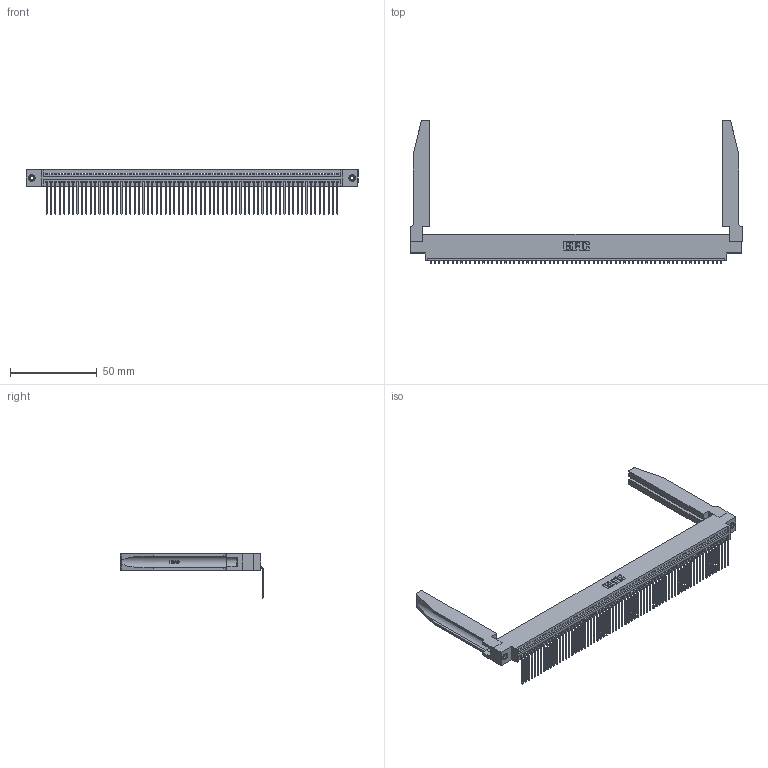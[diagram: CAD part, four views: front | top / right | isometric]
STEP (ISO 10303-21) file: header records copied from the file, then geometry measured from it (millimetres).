
FILE_DESCRIPTION (( 'STEP AP203' ), '1' );
FILE_NAME ('345-067-559-678.STEP', '2019-10-12T03:43:56', ( '' ), ( '' ), 'SwSTEP 2.0', 'SolidWorks 2016', '' );
FILE_SCHEMA (( 'CONFIG_CONTROL_DESIGN' ));
Length unit declared in the file: inch
Products named in the file (5): 345-292-001_558 559 Tail - 1; 345 Part_0.170 Offset - 0.156 Dia-TH; 345-250-001_345-250-001-102; 345-067-559-678; 345-220-078_345-220-078
Assembly tree (72 placements, depth 2):
  345-067-559-678
    345 Part_0.170 Offset - 0.156 Dia-TH
    345-292-001_558 559 Tail - 1  x67
    345-250-001_345-250-001-102  x2
    345-220-078_345-220-078  x2
Bounding box: 191.41 x 82.03 x 25.53 mm (x, y, z)
Volume: 26265.9 mm3; surface area: 33202.3 mm2
Topology: 72 solids, 72 shells, 4384 faces, 13155 edges, 8670 vertices
Faces by surface type: plane 3040, cylinder 1292, bspline 36, cone 12, torus 4
Entity records: 52016 total; most frequent: CARTESIAN_POINT 9908, ORIENTED_EDGE 8806, DIRECTION 7623, EDGE_CURVE 4403, LINE 3909, VECTOR 3909, VERTEX_POINT 2928, AXIS2_PLACEMENT_3D 1857
